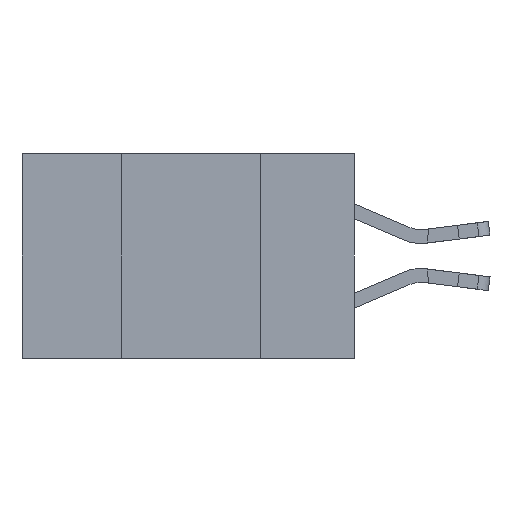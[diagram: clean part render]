
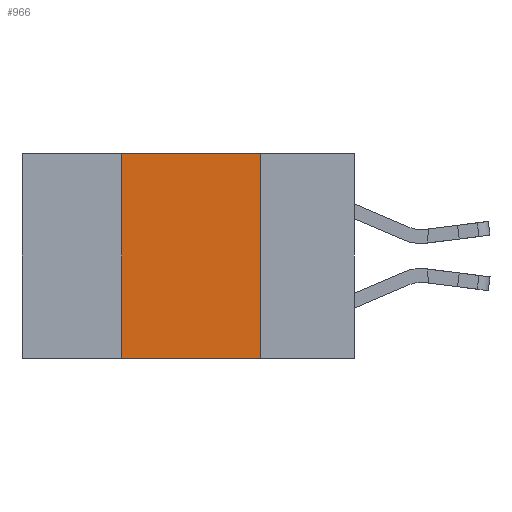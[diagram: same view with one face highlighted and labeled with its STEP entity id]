
A CAD part, left-side view. The second image highlights one B-rep face of the part: STEP entity #966.
In plain terms, the highlighted planar face has unit normal (-1, 0, 0).
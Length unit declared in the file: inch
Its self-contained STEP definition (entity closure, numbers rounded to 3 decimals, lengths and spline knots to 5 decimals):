
#28 = VERTEX_POINT ( 'NONE', #8497 ) ;
#601 = PLANE ( 'NONE',  #6499 ) ;
#618 = CARTESIAN_POINT ( 'NONE',  ( 0., 0.17, 0. ) ) ;
#675 = DIRECTION ( 'NONE',  ( 0., -1., 0. ) ) ;
#679 = CARTESIAN_POINT ( 'NONE',  ( 0., 0.6, 0. ) ) ;
#966 = ADVANCED_FACE ( 'NONE', ( #14510 ), #601, .F. ) ;
#1182 = CARTESIAN_POINT ( 'NONE',  ( 0., 0.6, 0. ) ) ;
#1564 = EDGE_LOOP ( 'NONE', ( #16643, #11697, #16108, #15357 ) ) ;
#1798 = VECTOR ( 'NONE', #21419, 39.37008 ) ;
#2061 = EDGE_CURVE ( 'NONE', #28, #20545, #6335, .T. ) ;
#2629 = DIRECTION ( 'NONE',  ( 1., 0., 0. ) ) ;
#2929 = DIRECTION ( 'NONE',  ( 0., -1., 0. ) ) ;
#2963 = DIRECTION ( 'NONE',  ( 0., 0., -1. ) ) ;
#3800 = EDGE_CURVE ( 'NONE', #8507, #15260, #13371, .T. ) ;
#5287 = DIRECTION ( 'NONE',  ( 0., 0., -1. ) ) ;
#6335 = LINE ( 'NONE', #21236, #1798 ) ;
#6499 = AXIS2_PLACEMENT_3D ( 'NONE', #679, #2629, #2963 ) ;
#6894 = CARTESIAN_POINT ( 'NONE',  ( 0., 0.17, -0.37 ) ) ;
#8497 = CARTESIAN_POINT ( 'NONE',  ( 0., 0.42, -0.37 ) ) ;
#8507 = VERTEX_POINT ( 'NONE', #618 ) ;
#9186 = CARTESIAN_POINT ( 'NONE',  ( 0., 0.6, -0.37 ) ) ;
#11697 = ORIENTED_EDGE ( 'NONE', *, *, #21330, .F. ) ;
#12750 = CARTESIAN_POINT ( 'NONE',  ( 0., 0.17, -0.37 ) ) ;
#13371 = LINE ( 'NONE', #12750, #17258 ) ;
#14510 = FACE_OUTER_BOUND ( 'NONE', #1564, .T. ) ;
#14549 = LINE ( 'NONE', #1182, #19006 ) ;
#15260 = VERTEX_POINT ( 'NONE', #6894 ) ;
#15357 = ORIENTED_EDGE ( 'NONE', *, *, #17850, .T. ) ;
#16090 = LINE ( 'NONE', #9186, #20033 ) ;
#16108 = ORIENTED_EDGE ( 'NONE', *, *, #2061, .F. ) ;
#16190 = CARTESIAN_POINT ( 'NONE',  ( 0., 0.42, 0. ) ) ;
#16643 = ORIENTED_EDGE ( 'NONE', *, *, #3800, .F. ) ;
#17258 = VECTOR ( 'NONE', #5287, 39.37008 ) ;
#17850 = EDGE_CURVE ( 'NONE', #28, #15260, #16090, .T. ) ;
#19006 = VECTOR ( 'NONE', #2929, 39.37008 ) ;
#20033 = VECTOR ( 'NONE', #675, 39.37008 ) ;
#20545 = VERTEX_POINT ( 'NONE', #16190 ) ;
#21236 = CARTESIAN_POINT ( 'NONE',  ( 0., 0.42, -0.37 ) ) ;
#21330 = EDGE_CURVE ( 'NONE', #20545, #8507, #14549, .T. ) ;
#21419 = DIRECTION ( 'NONE',  ( 0., 0., 1. ) ) ;
